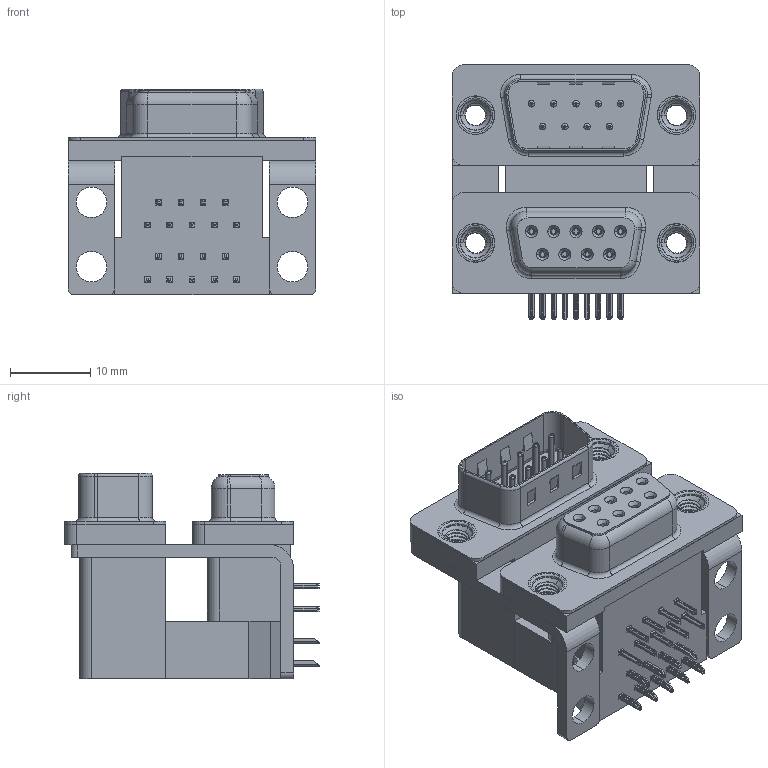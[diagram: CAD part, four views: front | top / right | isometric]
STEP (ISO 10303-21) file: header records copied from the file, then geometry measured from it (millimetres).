
FILE_DESCRIPTION (( 'STEP AP203' ), '1' );
FILE_NAME ('663-009-264-001.STEP', '2022-06-17T20:56:27', ( '' ), ( '' ), 'SwSTEP 2.0', 'SolidWorks 2020', '' );
FILE_SCHEMA (( 'CONFIG_CONTROL_DESIGN' ));
Length unit declared in the file: millimetre
Products named in the file (12): 663 Housing Lower_09 Contacts; 663 Contact Top Upper_L; 663 Housing Spacer_09 Contacts L; 663 Contact Bottom Upper_L; 663 Contact Bottom Lower; 663 Contact Top Lower; 663-009-264-001; 663 Threaded Rivet_M3; 663 Shell Receptacle_09 Contacts; 663 Mounting Bracket_NoneL; 663 Shell Plug_09 Contacts; 663 Housing Upper_09 Contacts L
Assembly tree (29 placements, depth 2):
  663-009-264-001
    663 Housing Lower_09 Contacts
    663 Housing Spacer_09 Contacts L
    663 Housing Upper_09 Contacts L
    663 Shell Receptacle_09 Contacts
    663 Shell Plug_09 Contacts
    663 Contact Bottom Lower  x4
    663 Contact Top Lower  x5
    663 Contact Bottom Upper_L  x4
    663 Contact Top Upper_L  x5
    663 Mounting Bracket_NoneL  x2
    663 Threaded Rivet_M3  x4
Bounding box: 30.81 x 31.61 x 25.6 mm (x, y, z)
Volume: 10331.7 mm3; surface area: 12032.9 mm2
Topology: 29 solids, 29 shells, 2533 faces, 6483 edges, 4057 vertices
Faces by surface type: plane 1263, cylinder 703, bspline 320, cone 124, torus 123
Entity records: 37150 total; most frequent: CARTESIAN_POINT 10822, ORIENTED_EDGE 5202, DIRECTION 4892, EDGE_CURVE 2601, LINE 1678, VECTOR 1678, VERTEX_POINT 1651, AXIS2_PLACEMENT_3D 1607
